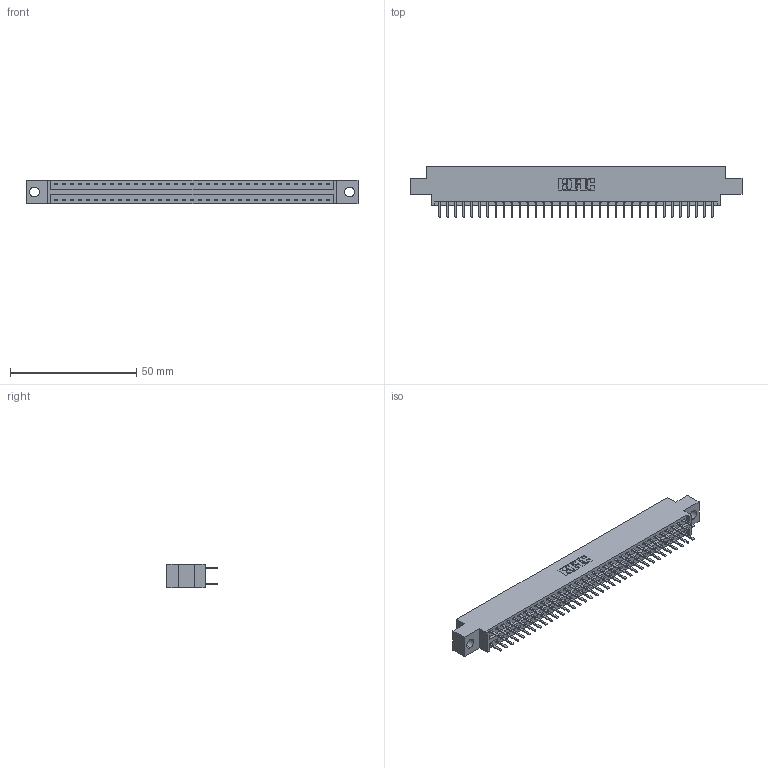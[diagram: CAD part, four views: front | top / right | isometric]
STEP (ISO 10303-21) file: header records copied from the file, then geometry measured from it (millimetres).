
FILE_DESCRIPTION (( 'STEP AP203' ), '1' );
FILE_NAME ('346-070-520-804.STEP', '2018-08-28T22:54:31', ( '' ), ( '' ), 'SwSTEP 2.0', 'SolidWorks 2016', '' );
FILE_SCHEMA (( 'CONFIG_CONTROL_DESIGN' ));
Length unit declared in the file: inch
Products named in the file (3): 346 Part_0.170 Offset - 0.156 Dia-TH; 345-292-001_345-293-120; 346-070-520-804
Assembly tree (71 placements, depth 2):
  346-070-520-804
    346 Part_0.170 Offset - 0.156 Dia-TH
    345-292-001_345-293-120  x70
Bounding box: 131.7 x 20.02 x 9.4 mm (x, y, z)
Volume: 12514.7 mm3; surface area: 17013.1 mm2
Topology: 71 solids, 71 shells, 4046 faces, 11751 edges, 7646 vertices
Faces by surface type: plane 2670, cylinder 1376
Entity records: 24033 total; most frequent: CARTESIAN_POINT 3984, ORIENTED_EDGE 3906, DIRECTION 3549, EDGE_CURVE 1953, LINE 1677, VECTOR 1677, VERTEX_POINT 1298, AXIS2_PLACEMENT_3D 936
